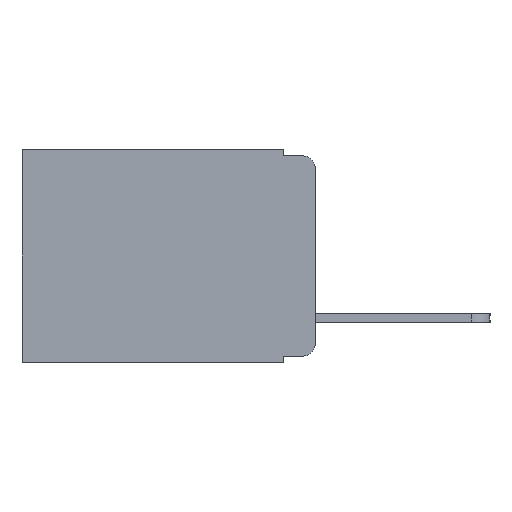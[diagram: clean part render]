
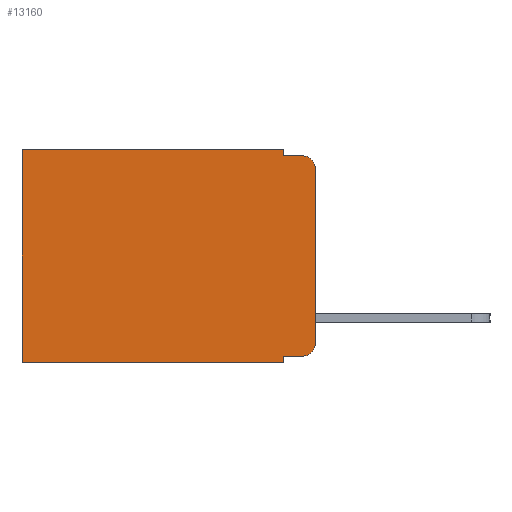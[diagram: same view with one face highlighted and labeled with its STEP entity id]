
A CAD part, left-side view. The second image highlights one B-rep face of the part: STEP entity #13160.
In plain terms, the highlighted planar face has unit normal (-1, 0, 0).
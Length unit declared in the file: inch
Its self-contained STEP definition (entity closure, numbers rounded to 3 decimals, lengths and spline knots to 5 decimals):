
#243 = DIRECTION ( 'NONE',  ( 0., -1., 0. ) ) ;
#254 = VERTEX_POINT ( 'NONE', #3049 ) ;
#421 = LINE ( 'NONE', #8570, #12398 ) ;
#596 = AXIS2_PLACEMENT_3D ( 'NONE', #2673, #10666, #3831 ) ;
#658 = ORIENTED_EDGE ( 'NONE', *, *, #10136, .F. ) ;
#853 = ORIENTED_EDGE ( 'NONE', *, *, #11376, .T. ) ;
#896 = VERTEX_POINT ( 'NONE', #2848 ) ;
#1009 = EDGE_LOOP ( 'NONE', ( #2052, #1662, #1979, #658, #12774, #5593, #5718, #4891, #6549, #853 ) ) ;
#1182 = VERTEX_POINT ( 'NONE', #8313 ) ;
#1244 = CARTESIAN_POINT ( 'NONE',  ( 0.298, 0., 0. ) ) ;
#1566 = DIRECTION ( 'NONE',  ( -1., 0., 0. ) ) ;
#1662 = ORIENTED_EDGE ( 'NONE', *, *, #10785, .T. ) ;
#1979 = ORIENTED_EDGE ( 'NONE', *, *, #7117, .F. ) ;
#2052 = ORIENTED_EDGE ( 'NONE', *, *, #7948, .F. ) ;
#2178 = VERTEX_POINT ( 'NONE', #12228 ) ;
#2354 = LINE ( 'NONE', #11059, #11475 ) ;
#2622 = VECTOR ( 'NONE', #4245, 39.37008 ) ;
#2673 = CARTESIAN_POINT ( 'NONE',  ( 0.298, 0.02, -0.313 ) ) ;
#2848 = CARTESIAN_POINT ( 'NONE',  ( 0.298, 0.051, -0.01 ) ) ;
#2912 = CARTESIAN_POINT ( 'NONE',  ( 0.298, 0.02, -0.333 ) ) ;
#3049 = CARTESIAN_POINT ( 'NONE',  ( 0.298, 0.051, 0. ) ) ;
#3050 = CIRCLE ( 'NONE', #596, 0.02 ) ;
#3116 = EDGE_CURVE ( 'NONE', #13439, #11525, #421, .T. ) ;
#3243 = DIRECTION ( 'NONE',  ( 1., 0., 0. ) ) ;
#3267 = DIRECTION ( 'NONE',  ( 0., 0., -1. ) ) ;
#3605 = CARTESIAN_POINT ( 'NONE',  ( 0.298, 0., -0.313 ) ) ;
#3694 = CARTESIAN_POINT ( 'NONE',  ( 0.298, 0., -0.03 ) ) ;
#3831 = DIRECTION ( 'NONE',  ( 0., 0., -1. ) ) ;
#3881 = CARTESIAN_POINT ( 'NONE',  ( 0.298, 0.051, -0.01 ) ) ;
#4052 = CARTESIAN_POINT ( 'NONE',  ( 0.298, 0.051, 0. ) ) ;
#4143 = AXIS2_PLACEMENT_3D ( 'NONE', #13388, #3243, #11209 ) ;
#4245 = DIRECTION ( 'NONE',  ( 0., 0., -1. ) ) ;
#4353 = CARTESIAN_POINT ( 'NONE',  ( 0.298, 0.473, 0. ) ) ;
#4401 = LINE ( 'NONE', #4052, #10508 ) ;
#4784 = EDGE_CURVE ( 'NONE', #10582, #2178, #7428, .T. ) ;
#4843 = DIRECTION ( 'NONE',  ( 0., 1., 0. ) ) ;
#4891 = ORIENTED_EDGE ( 'NONE', *, *, #7827, .F. ) ;
#4921 = CARTESIAN_POINT ( 'NONE',  ( 0.298, 0., -0.343 ) ) ;
#4972 = VECTOR ( 'NONE', #5900, 39.37008 ) ;
#5246 = LINE ( 'NONE', #3881, #8017 ) ;
#5308 = CARTESIAN_POINT ( 'NONE',  ( 0.298, 0., 0. ) ) ;
#5336 = CARTESIAN_POINT ( 'NONE',  ( 0.298, 0.02, -0.01 ) ) ;
#5593 = ORIENTED_EDGE ( 'NONE', *, *, #11660, .T. ) ;
#5718 = ORIENTED_EDGE ( 'NONE', *, *, #4784, .F. ) ;
#5900 = DIRECTION ( 'NONE',  ( 0., 1., 0. ) ) ;
#5960 = VERTEX_POINT ( 'NONE', #3605 ) ;
#6549 = ORIENTED_EDGE ( 'NONE', *, *, #3116, .T. ) ;
#7117 = EDGE_CURVE ( 'NONE', #896, #13654, #5246, .T. ) ;
#7171 = VECTOR ( 'NONE', #3267, 39.37008 ) ;
#7390 = CIRCLE ( 'NONE', #12786, 0.02 ) ;
#7428 = LINE ( 'NONE', #4921, #13042 ) ;
#7827 = EDGE_CURVE ( 'NONE', #13439, #10582, #4401, .T. ) ;
#7948 = EDGE_CURVE ( 'NONE', #8335, #5960, #9468, .T. ) ;
#8017 = VECTOR ( 'NONE', #243, 39.37008 ) ;
#8097 = LINE ( 'NONE', #1244, #4972 ) ;
#8293 = CARTESIAN_POINT ( 'NONE',  ( 0.298, 0.051, -0.343 ) ) ;
#8313 = CARTESIAN_POINT ( 'NONE',  ( 0.298, 0.473, 0. ) ) ;
#8335 = VERTEX_POINT ( 'NONE', #3694 ) ;
#8544 = CARTESIAN_POINT ( 'NONE',  ( 0.298, 0.02, -0.03 ) ) ;
#8570 = CARTESIAN_POINT ( 'NONE',  ( 0.298, 0.051, -0.333 ) ) ;
#9468 = LINE ( 'NONE', #5308, #2622 ) ;
#9499 = FACE_OUTER_BOUND ( 'NONE', #1009, .T. ) ;
#9733 = DIRECTION ( 'NONE',  ( 0., 0., -1. ) ) ;
#10136 = EDGE_CURVE ( 'NONE', #254, #896, #2354, .T. ) ;
#10380 = DIRECTION ( 'NONE',  ( 0., -1., 0. ) ) ;
#10508 = VECTOR ( 'NONE', #10885, 39.37008 ) ;
#10582 = VERTEX_POINT ( 'NONE', #8293 ) ;
#10666 = DIRECTION ( 'NONE',  ( -1., 0., 0. ) ) ;
#10785 = EDGE_CURVE ( 'NONE', #8335, #13654, #7390, .T. ) ;
#10885 = DIRECTION ( 'NONE',  ( 0., 0., -1. ) ) ;
#11059 = CARTESIAN_POINT ( 'NONE',  ( 0.298, 0.051, 0. ) ) ;
#11209 = DIRECTION ( 'NONE',  ( 0., 0., -1. ) ) ;
#11376 = EDGE_CURVE ( 'NONE', #11525, #5960, #3050, .T. ) ;
#11475 = VECTOR ( 'NONE', #14455, 39.37008 ) ;
#11525 = VERTEX_POINT ( 'NONE', #2912 ) ;
#11660 = EDGE_CURVE ( 'NONE', #1182, #2178, #13496, .T. ) ;
#12228 = CARTESIAN_POINT ( 'NONE',  ( 0.298, 0.473, -0.343 ) ) ;
#12398 = VECTOR ( 'NONE', #10380, 39.37008 ) ;
#12774 = ORIENTED_EDGE ( 'NONE', *, *, #13398, .T. ) ;
#12786 = AXIS2_PLACEMENT_3D ( 'NONE', #8544, #1566, #9733 ) ;
#13042 = VECTOR ( 'NONE', #4843, 39.37008 ) ;
#13160 = ADVANCED_FACE ( 'NONE', ( #9499 ), #14550, .F. ) ;
#13388 = CARTESIAN_POINT ( 'NONE',  ( 0.298, 0., 0. ) ) ;
#13398 = EDGE_CURVE ( 'NONE', #254, #1182, #8097, .T. ) ;
#13439 = VERTEX_POINT ( 'NONE', #14037 ) ;
#13496 = LINE ( 'NONE', #4353, #7171 ) ;
#13654 = VERTEX_POINT ( 'NONE', #5336 ) ;
#14037 = CARTESIAN_POINT ( 'NONE',  ( 0.298, 0.051, -0.333 ) ) ;
#14455 = DIRECTION ( 'NONE',  ( 0., 0., -1. ) ) ;
#14550 = PLANE ( 'NONE',  #4143 ) ;
